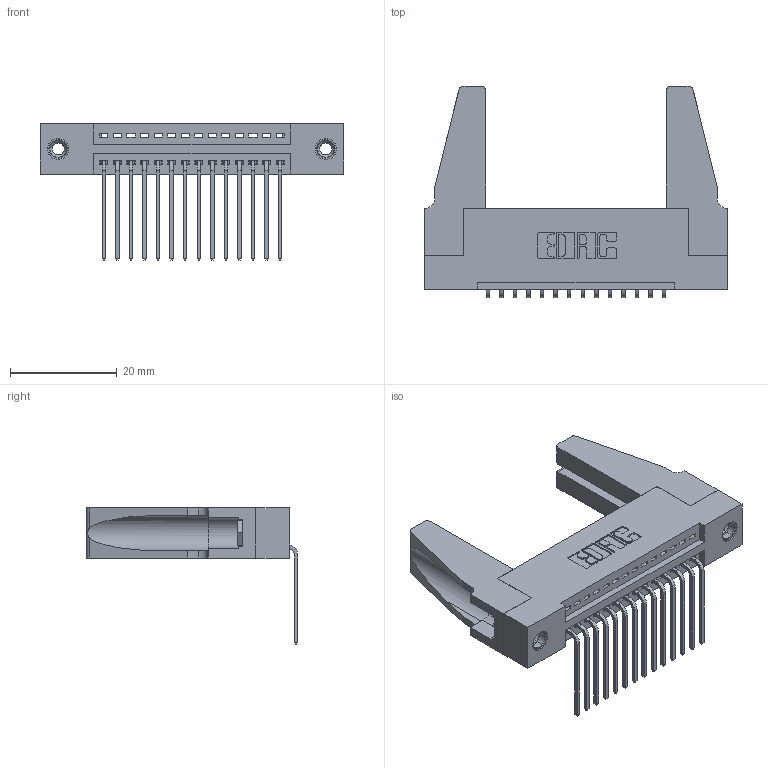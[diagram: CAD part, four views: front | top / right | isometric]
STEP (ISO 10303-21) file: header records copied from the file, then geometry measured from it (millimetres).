
FILE_DESCRIPTION (( 'STEP AP203' ), '1' );
FILE_NAME ('395-014-559-188.STEP', '2019-10-16T05:29:06', ( '' ), ( '' ), 'SwSTEP 2.0', 'SolidWorks 2016', '' );
FILE_SCHEMA (( 'CONFIG_CONTROL_DESIGN' ));
Length unit declared in the file: inch
Products named in the file (5): 345-292-001_558 559 Tail - 1; 345-250-001_345-250-001-102; 345-220-078_345-220-088; 345 Part_Flush Mounting Lugs - 0.156 Dia-TH; 395-014-559-188
Assembly tree (19 placements, depth 2):
  395-014-559-188
    345 Part_Flush Mounting Lugs - 0.156 Dia-TH
    345-292-001_558 559 Tail - 1  x14
    345-250-001_345-250-001-102  x2
    345-220-078_345-220-088  x2
Bounding box: 56.79 x 39.61 x 25.53 mm (x, y, z)
Volume: 8464.2 mm3; surface area: 9948.6 mm2
Topology: 19 solids, 19 shells, 1090 faces, 3203 edges, 2106 vertices
Faces by surface type: plane 740, cylinder 334, cone 12, torus 4
Entity records: 16538 total; most frequent: CARTESIAN_POINT 2856, ORIENTED_EDGE 2764, DIRECTION 2542, EDGE_CURVE 1382, VECTOR 1152, LINE 1152, VERTEX_POINT 914, AXIS2_PLACEMENT_3D 695
